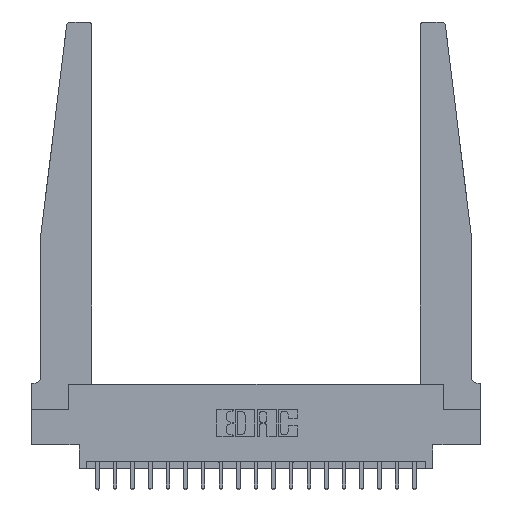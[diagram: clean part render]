
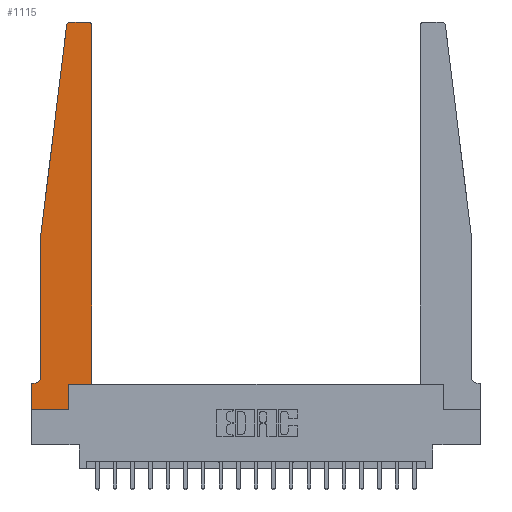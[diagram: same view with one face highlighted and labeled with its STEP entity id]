
A CAD part, top view. The second image highlights one B-rep face of the part: STEP entity #1115.
In plain terms, the highlighted planar face has unit normal (0, 0, 1).
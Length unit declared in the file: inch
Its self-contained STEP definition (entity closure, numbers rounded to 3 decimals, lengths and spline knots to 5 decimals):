
#82 = ORIENTED_EDGE ( 'NONE', *, *, #8455, .T. ) ;
#135 = ORIENTED_EDGE ( 'NONE', *, *, #1522, .T. ) ;
#371 = VECTOR ( 'NONE', #8792, 39.37008 ) ;
#499 = VECTOR ( 'NONE', #11269, 39.37008 ) ;
#648 = EDGE_LOOP ( 'NONE', ( #1034, #5141, #19088, #10962, #18485, #11664, #82, #8165, #135, #17697, #15240, #1209 ) ) ;
#843 = DIRECTION ( 'NONE',  ( 1., 0., 0. ) ) ;
#1034 = ORIENTED_EDGE ( 'NONE', *, *, #18066, .T. ) ;
#1068 = CARTESIAN_POINT ( 'NONE',  ( 0.065, 1.25, 0.37 ) ) ;
#1115 = ADVANCED_FACE ( 'NONE', ( #11790 ), #4688, .T. ) ;
#1209 = ORIENTED_EDGE ( 'NONE', *, *, #17440, .T. ) ;
#1214 = DIRECTION ( 'NONE',  ( -1., 0., 0. ) ) ;
#1313 = VERTEX_POINT ( 'NONE', #13038 ) ;
#1368 = CIRCLE ( 'NONE', #4898, 0.03 ) ;
#1522 = EDGE_CURVE ( 'NONE', #1313, #18450, #1687, .T. ) ;
#1667 = CARTESIAN_POINT ( 'NONE',  ( 0.425, 0.18, 0.37 ) ) ;
#1687 = LINE ( 'NONE', #4402, #5408 ) ;
#1911 = VERTEX_POINT ( 'NONE', #13167 ) ;
#2235 = VECTOR ( 'NONE', #8947, 39.37008 ) ;
#2249 = CARTESIAN_POINT ( 'NONE',  ( 0.065, 0.2375, 0.37 ) ) ;
#2336 = CARTESIAN_POINT ( 'NONE',  ( 0.24675, 2.72367, 0.37 ) ) ;
#2574 = VERTEX_POINT ( 'NONE', #13216 ) ;
#2744 = DIRECTION ( 'NONE',  ( 0., 0., 1. ) ) ;
#2906 = DIRECTION ( 'NONE',  ( 0., 1., 0. ) ) ;
#3449 = CARTESIAN_POINT ( 'NONE',  ( 0., 0., 0.37 ) ) ;
#3914 = VERTEX_POINT ( 'NONE', #7327 ) ;
#4156 = CARTESIAN_POINT ( 'NONE',  ( 0.065, 0.1875, 0.37 ) ) ;
#4402 = CARTESIAN_POINT ( 'NONE',  ( 0.2605, 0.18, 0.37 ) ) ;
#4490 = VERTEX_POINT ( 'NONE', #2336 ) ;
#4514 = CARTESIAN_POINT ( 'NONE',  ( 0.425, 0.18, 0.37 ) ) ;
#4574 = CARTESIAN_POINT ( 'NONE',  ( 0.015, 0.1875, 0.37 ) ) ;
#4688 = PLANE ( 'NONE',  #13798 ) ;
#4898 = AXIS2_PLACEMENT_3D ( 'NONE', #19744, #10292, #843 ) ;
#5080 = VERTEX_POINT ( 'NONE', #2249 ) ;
#5141 = ORIENTED_EDGE ( 'NONE', *, *, #10753, .T. ) ;
#5408 = VECTOR ( 'NONE', #2906, 39.37008 ) ;
#5607 = DIRECTION ( 'NONE',  ( 0., 0., -1. ) ) ;
#5624 = CARTESIAN_POINT ( 'NONE',  ( 0.425, 0.18, 0.37 ) ) ;
#7302 = LINE ( 'NONE', #10716, #10951 ) ;
#7327 = CARTESIAN_POINT ( 'NONE',  ( 0.065, 1.25, 0.37 ) ) ;
#7366 = EDGE_CURVE ( 'NONE', #18450, #15262, #11153, .T. ) ;
#7583 = AXIS2_PLACEMENT_3D ( 'NONE', #15017, #5607, #16594 ) ;
#7888 = CARTESIAN_POINT ( 'NONE',  ( 0., 0.1875, 0.37 ) ) ;
#8165 = ORIENTED_EDGE ( 'NONE', *, *, #14561, .T. ) ;
#8197 = VECTOR ( 'NONE', #9149, 39.37008 ) ;
#8455 = EDGE_CURVE ( 'NONE', #17583, #15110, #12315, .T. ) ;
#8532 = VERTEX_POINT ( 'NONE', #4574 ) ;
#8604 = CARTESIAN_POINT ( 'NONE',  ( 0.2605, 0.18, 0.37 ) ) ;
#8706 = LINE ( 'NONE', #18733, #16552 ) ;
#8792 = DIRECTION ( 'NONE',  ( 0., 1., 0. ) ) ;
#8908 = LINE ( 'NONE', #3449, #499 ) ;
#8947 = DIRECTION ( 'NONE',  ( -0.122, -0.992, 0. ) ) ;
#9149 = DIRECTION ( 'NONE',  ( 0., -1., 0. ) ) ;
#9344 = CIRCLE ( 'NONE', #12048, 0.03 ) ;
#9450 = DIRECTION ( 'NONE',  ( 1., 0., 0. ) ) ;
#9528 = DIRECTION ( 'NONE',  ( 1., 0., 0. ) ) ;
#10292 = DIRECTION ( 'NONE',  ( 0., 0., 1. ) ) ;
#10716 = CARTESIAN_POINT ( 'NONE',  ( 0.25, 2.75, 0.37 ) ) ;
#10753 = EDGE_CURVE ( 'NONE', #2574, #4490, #9344, .T. ) ;
#10951 = VECTOR ( 'NONE', #1214, 39.37008 ) ;
#10962 = ORIENTED_EDGE ( 'NONE', *, *, #12533, .T. ) ;
#10975 = CARTESIAN_POINT ( 'NONE',  ( 0.395, 2.75, 0.37 ) ) ;
#11153 = LINE ( 'NONE', #1667, #15339 ) ;
#11269 = DIRECTION ( 'NONE',  ( 1., 0., 0. ) ) ;
#11664 = ORIENTED_EDGE ( 'NONE', *, *, #13665, .T. ) ;
#11790 = FACE_OUTER_BOUND ( 'NONE', #648, .T. ) ;
#12048 = AXIS2_PLACEMENT_3D ( 'NONE', #12126, #2744, #13719 ) ;
#12126 = CARTESIAN_POINT ( 'NONE',  ( 0.27653, 2.72, 0.37 ) ) ;
#12315 = LINE ( 'NONE', #20092, #8197 ) ;
#12422 = DIRECTION ( 'NONE',  ( 0., -1., 0. ) ) ;
#12533 = EDGE_CURVE ( 'NONE', #3914, #5080, #8706, .T. ) ;
#13038 = CARTESIAN_POINT ( 'NONE',  ( 0.2605, 0., 0.37 ) ) ;
#13167 = CARTESIAN_POINT ( 'NONE',  ( 0.425, 2.72, 0.37 ) ) ;
#13216 = CARTESIAN_POINT ( 'NONE',  ( 0.27653, 2.75, 0.37 ) ) ;
#13665 = EDGE_CURVE ( 'NONE', #8532, #17583, #14824, .T. ) ;
#13719 = DIRECTION ( 'NONE',  ( 1., 0., 0. ) ) ;
#13798 = AXIS2_PLACEMENT_3D ( 'NONE', #7888, #18889, #9450 ) ;
#14561 = EDGE_CURVE ( 'NONE', #15110, #1313, #8908, .T. ) ;
#14764 = LINE ( 'NONE', #1068, #2235 ) ;
#14824 = LINE ( 'NONE', #4156, #18528 ) ;
#15017 = CARTESIAN_POINT ( 'NONE',  ( 0.015, 0.2375, 0.37 ) ) ;
#15110 = VERTEX_POINT ( 'NONE', #19899 ) ;
#15171 = EDGE_CURVE ( 'NONE', #4490, #3914, #14764, .T. ) ;
#15240 = ORIENTED_EDGE ( 'NONE', *, *, #17462, .T. ) ;
#15262 = VERTEX_POINT ( 'NONE', #4514 ) ;
#15339 = VECTOR ( 'NONE', #9528, 39.37008 ) ;
#15343 = VERTEX_POINT ( 'NONE', #10975 ) ;
#16552 = VECTOR ( 'NONE', #12422, 39.37008 ) ;
#16594 = DIRECTION ( 'NONE',  ( -1., 0., 0. ) ) ;
#16816 = CARTESIAN_POINT ( 'NONE',  ( 0., 0.1875, 0.37 ) ) ;
#17132 = LINE ( 'NONE', #5624, #371 ) ;
#17440 = EDGE_CURVE ( 'NONE', #1911, #15343, #1368, .T. ) ;
#17462 = EDGE_CURVE ( 'NONE', #15262, #1911, #17132, .T. ) ;
#17583 = VERTEX_POINT ( 'NONE', #16816 ) ;
#17697 = ORIENTED_EDGE ( 'NONE', *, *, #7366, .T. ) ;
#18066 = EDGE_CURVE ( 'NONE', #15343, #2574, #7302, .T. ) ;
#18331 = DIRECTION ( 'NONE',  ( -1., 0., 0. ) ) ;
#18450 = VERTEX_POINT ( 'NONE', #8604 ) ;
#18485 = ORIENTED_EDGE ( 'NONE', *, *, #19036, .T. ) ;
#18528 = VECTOR ( 'NONE', #18331, 39.37008 ) ;
#18733 = CARTESIAN_POINT ( 'NONE',  ( 0.065, 1.25, 0.37 ) ) ;
#18889 = DIRECTION ( 'NONE',  ( 0., 0., 1. ) ) ;
#19036 = EDGE_CURVE ( 'NONE', #5080, #8532, #20215, .T. ) ;
#19088 = ORIENTED_EDGE ( 'NONE', *, *, #15171, .T. ) ;
#19744 = CARTESIAN_POINT ( 'NONE',  ( 0.395, 2.72, 0.37 ) ) ;
#19899 = CARTESIAN_POINT ( 'NONE',  ( 0., 0., 0.37 ) ) ;
#20092 = CARTESIAN_POINT ( 'NONE',  ( 0., 0., 0.37 ) ) ;
#20215 = CIRCLE ( 'NONE', #7583, 0.05 ) ;
